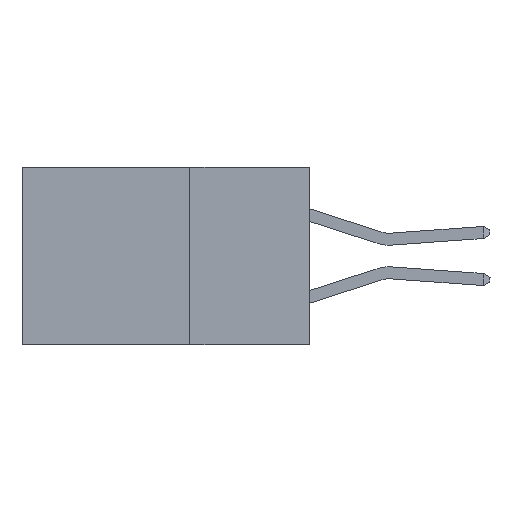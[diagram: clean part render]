
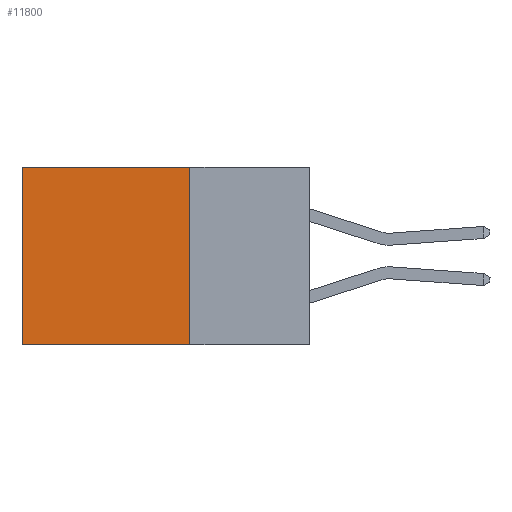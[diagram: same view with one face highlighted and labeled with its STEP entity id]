
A CAD part, left-side view. The second image highlights one B-rep face of the part: STEP entity #11800.
In plain terms, the highlighted planar face has unit normal (-1, 0, 0).
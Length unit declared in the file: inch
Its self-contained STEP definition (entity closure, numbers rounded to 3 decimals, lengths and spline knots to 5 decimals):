
#188 = VERTEX_POINT ( 'NONE', #18461 ) ;
#293 = CARTESIAN_POINT ( 'NONE',  ( 0.2615, 0.25, -0.37 ) ) ;
#964 = EDGE_CURVE ( 'NONE', #5477, #188, #1416, .T. ) ;
#1416 = LINE ( 'NONE', #15366, #14389 ) ;
#2133 = AXIS2_PLACEMENT_3D ( 'NONE', #4295, #15637, #5931 ) ;
#3361 = ORIENTED_EDGE ( 'NONE', *, *, #19685, .T. ) ;
#3434 = VECTOR ( 'NONE', #7391, 39.37008 ) ;
#4295 = CARTESIAN_POINT ( 'NONE',  ( 0.2615, 0.25, -0.37 ) ) ;
#4532 = LINE ( 'NONE', #293, #7838 ) ;
#4789 = CARTESIAN_POINT ( 'NONE',  ( 0.2615, 0.6, -0.37 ) ) ;
#5252 = VERTEX_POINT ( 'NONE', #8457 ) ;
#5477 = VERTEX_POINT ( 'NONE', #15507 ) ;
#5931 = DIRECTION ( 'NONE',  ( 0., 0., -1. ) ) ;
#6775 = DIRECTION ( 'NONE',  ( 0., 0., -1. ) ) ;
#7391 = DIRECTION ( 'NONE',  ( 0., 1., 0. ) ) ;
#7561 = ORIENTED_EDGE ( 'NONE', *, *, #12207, .F. ) ;
#7838 = VECTOR ( 'NONE', #6775, 39.37008 ) ;
#8457 = CARTESIAN_POINT ( 'NONE',  ( 0.2615, 0.25, 0. ) ) ;
#8952 = CARTESIAN_POINT ( 'NONE',  ( 0.2615, 0.25, 0. ) ) ;
#9402 = EDGE_LOOP ( 'NONE', ( #18948, #20800, #7561, #3361 ) ) ;
#10415 = DIRECTION ( 'NONE',  ( 0., 1., 0. ) ) ;
#11187 = FACE_OUTER_BOUND ( 'NONE', #9402, .T. ) ;
#11800 = ADVANCED_FACE ( 'NONE', ( #11187 ), #18883, .F. ) ;
#12103 = LINE ( 'NONE', #8952, #3434 ) ;
#12207 = EDGE_CURVE ( 'NONE', #5252, #5477, #4532, .T. ) ;
#13145 = LINE ( 'NONE', #4789, #17427 ) ;
#14389 = VECTOR ( 'NONE', #10415, 39.37008 ) ;
#15292 = VERTEX_POINT ( 'NONE', #19960 ) ;
#15366 = CARTESIAN_POINT ( 'NONE',  ( 0.2615, 0.25, -0.37 ) ) ;
#15507 = CARTESIAN_POINT ( 'NONE',  ( 0.2615, 0.25, -0.37 ) ) ;
#15637 = DIRECTION ( 'NONE',  ( 1., 0., 0. ) ) ;
#16121 = DIRECTION ( 'NONE',  ( 0., 0., -1. ) ) ;
#17427 = VECTOR ( 'NONE', #16121, 39.37008 ) ;
#18461 = CARTESIAN_POINT ( 'NONE',  ( 0.2615, 0.6, -0.37 ) ) ;
#18716 = EDGE_CURVE ( 'NONE', #15292, #188, #13145, .T. ) ;
#18883 = PLANE ( 'NONE',  #2133 ) ;
#18948 = ORIENTED_EDGE ( 'NONE', *, *, #18716, .T. ) ;
#19685 = EDGE_CURVE ( 'NONE', #5252, #15292, #12103, .T. ) ;
#19960 = CARTESIAN_POINT ( 'NONE',  ( 0.2615, 0.6, 0. ) ) ;
#20800 = ORIENTED_EDGE ( 'NONE', *, *, #964, .F. ) ;
